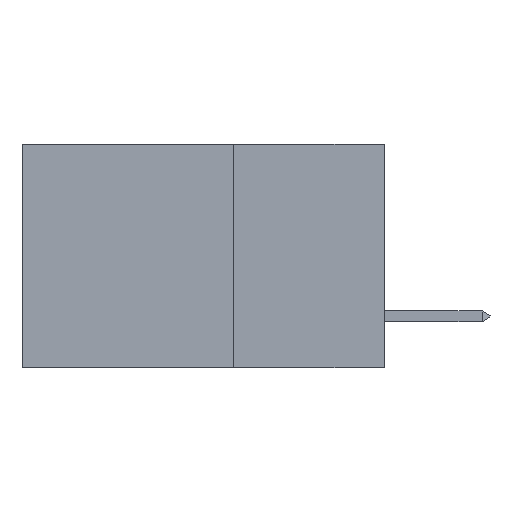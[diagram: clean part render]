
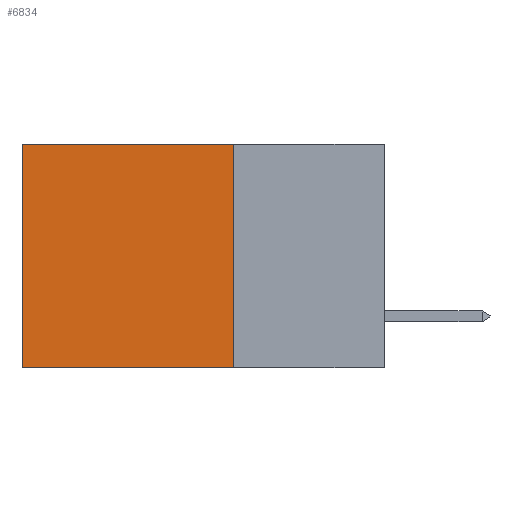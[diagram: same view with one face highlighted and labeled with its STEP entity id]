
A CAD part, left-side view. The second image highlights one B-rep face of the part: STEP entity #6834.
In plain terms, the highlighted planar face has unit normal (-1, 0, 0).
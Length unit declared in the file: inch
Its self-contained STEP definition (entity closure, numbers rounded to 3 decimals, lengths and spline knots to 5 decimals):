
#75 = VECTOR ( 'NONE', #2095, 39.37008 ) ;
#543 = VERTEX_POINT ( 'NONE', #5537 ) ;
#789 = VECTOR ( 'NONE', #2428, 39.37008 ) ;
#794 = CARTESIAN_POINT ( 'NONE',  ( 0.2875, 0.25, 0. ) ) ;
#845 = DIRECTION ( 'NONE',  ( 0., 0., -1. ) ) ;
#1258 = VERTEX_POINT ( 'NONE', #7309 ) ;
#1547 = PLANE ( 'NONE',  #2190 ) ;
#1676 = CARTESIAN_POINT ( 'NONE',  ( 0.2875, 0.6, 0. ) ) ;
#1700 = EDGE_CURVE ( 'NONE', #543, #2055, #6588, .T. ) ;
#1828 = VECTOR ( 'NONE', #6713, 39.37008 ) ;
#2055 = VERTEX_POINT ( 'NONE', #6436 ) ;
#2095 = DIRECTION ( 'NONE',  ( 0., 1., 0. ) ) ;
#2175 = ORIENTED_EDGE ( 'NONE', *, *, #3284, .F. ) ;
#2190 = AXIS2_PLACEMENT_3D ( 'NONE', #794, #3655, #845 ) ;
#2305 = DIRECTION ( 'NONE',  ( 0., 1., 0. ) ) ;
#2367 = ORIENTED_EDGE ( 'NONE', *, *, #8797, .F. ) ;
#2428 = DIRECTION ( 'NONE',  ( 0., 0., -1. ) ) ;
#2941 = CARTESIAN_POINT ( 'NONE',  ( 0.2875, 0.25, -0.37 ) ) ;
#3284 = EDGE_CURVE ( 'NONE', #543, #1258, #5252, .T. ) ;
#3655 = DIRECTION ( 'NONE',  ( 1., 0., 0. ) ) ;
#3703 = CARTESIAN_POINT ( 'NONE',  ( 0.2875, 0.25, 0. ) ) ;
#3764 = ORIENTED_EDGE ( 'NONE', *, *, #1700, .T. ) ;
#3879 = EDGE_CURVE ( 'NONE', #2055, #4646, #5915, .T. ) ;
#4201 = ORIENTED_EDGE ( 'NONE', *, *, #3879, .T. ) ;
#4646 = VERTEX_POINT ( 'NONE', #7202 ) ;
#5013 = LINE ( 'NONE', #2941, #75 ) ;
#5252 = LINE ( 'NONE', #3703, #1828 ) ;
#5537 = CARTESIAN_POINT ( 'NONE',  ( 0.2875, 0.25, 0. ) ) ;
#5915 = LINE ( 'NONE', #1676, #789 ) ;
#6436 = CARTESIAN_POINT ( 'NONE',  ( 0.2875, 0.6, 0. ) ) ;
#6588 = LINE ( 'NONE', #8734, #8116 ) ;
#6713 = DIRECTION ( 'NONE',  ( 0., 0., -1. ) ) ;
#6834 = ADVANCED_FACE ( 'NONE', ( #8675 ), #1547, .F. ) ;
#7202 = CARTESIAN_POINT ( 'NONE',  ( 0.2875, 0.6, -0.37 ) ) ;
#7309 = CARTESIAN_POINT ( 'NONE',  ( 0.2875, 0.25, -0.37 ) ) ;
#8116 = VECTOR ( 'NONE', #2305, 39.37008 ) ;
#8650 = EDGE_LOOP ( 'NONE', ( #4201, #2367, #2175, #3764 ) ) ;
#8675 = FACE_OUTER_BOUND ( 'NONE', #8650, .T. ) ;
#8734 = CARTESIAN_POINT ( 'NONE',  ( 0.2875, 0.25, 0. ) ) ;
#8797 = EDGE_CURVE ( 'NONE', #1258, #4646, #5013, .T. ) ;
